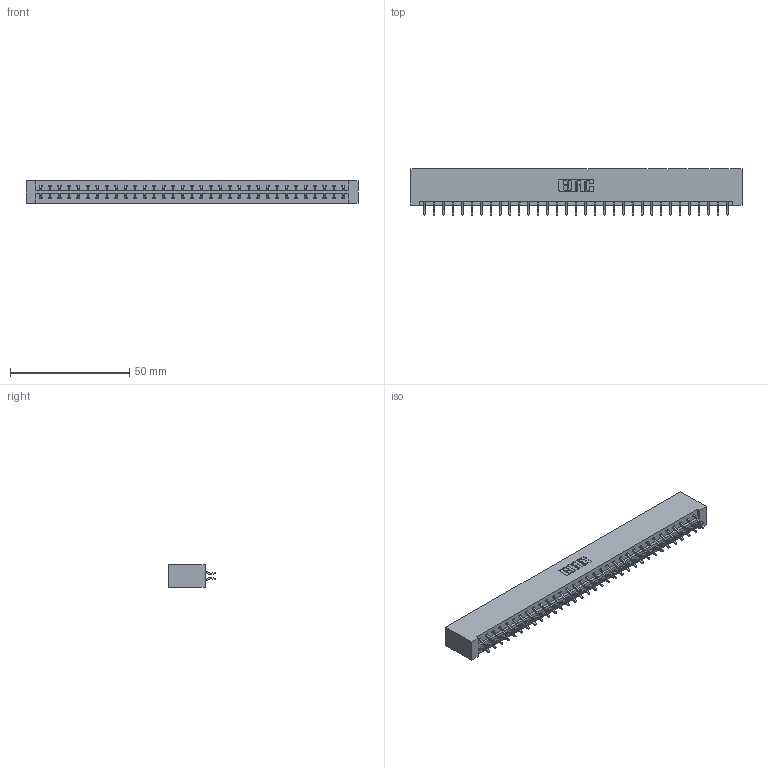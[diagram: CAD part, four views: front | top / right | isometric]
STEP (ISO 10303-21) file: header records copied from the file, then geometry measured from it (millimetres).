
FILE_DESCRIPTION (( 'STEP AP203' ), '1' );
FILE_NAME ('333-066-556-201.STEP', '2018-08-04T11:52:16', ( '' ), ( '' ), 'SwSTEP 2.0', 'SolidWorks 2016', '' );
FILE_SCHEMA (( 'CONFIG_CONTROL_DESIGN' ));
Length unit declared in the file: inch
Products named in the file (3): 333 Part_Lugless; 345-292-001_556 Tail; 333-066-556-201
Assembly tree (67 placements, depth 2):
  333-066-556-201
    333 Part_Lugless
    345-292-001_556 Tail  x66
Bounding box: 139.01 x 19.57 x 9.4 mm (x, y, z)
Volume: 14738 mm3; surface area: 17286.5 mm2
Topology: 67 solids, 67 shells, 3934 faces, 11705 edges, 7714 vertices
Faces by surface type: plane 2706, cylinder 1228
Entity records: 22337 total; most frequent: CARTESIAN_POINT 3726, ORIENTED_EDGE 3650, DIRECTION 3181, EDGE_CURVE 1825, VECTOR 1697, LINE 1697, VERTEX_POINT 1214, AXIS2_PLACEMENT_3D 742
